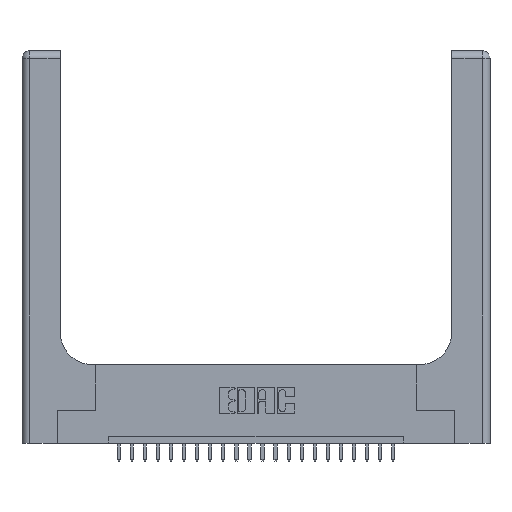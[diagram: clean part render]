
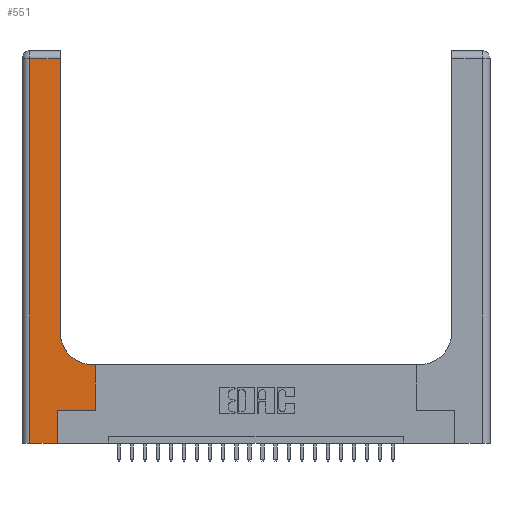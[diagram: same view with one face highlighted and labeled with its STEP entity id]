
A CAD part, top view. The second image highlights one B-rep face of the part: STEP entity #551.
In plain terms, the highlighted planar face has unit normal (0, 0, 1).
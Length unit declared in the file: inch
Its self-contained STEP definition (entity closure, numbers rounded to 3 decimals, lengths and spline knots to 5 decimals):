
#551 = ADVANCED_FACE ( 'NONE', ( #5901 ), #21168, .F. ) ;
#574 = ORIENTED_EDGE ( 'NONE', *, *, #9648, .T. ) ;
#747 = LINE ( 'NONE', #5997, #8378 ) ;
#786 = VECTOR ( 'NONE', #13788, 39.37008 ) ;
#1562 = EDGE_CURVE ( 'NONE', #21603, #2287, #7590, .T. ) ;
#2083 = VECTOR ( 'NONE', #13588, 39.37008 ) ;
#2287 = VERTEX_POINT ( 'NONE', #13245 ) ;
#2296 = DIRECTION ( 'NONE',  ( -1., 0., 0. ) ) ;
#2639 = CIRCLE ( 'NONE', #22379, 0.25 ) ;
#2671 = AXIS2_PLACEMENT_3D ( 'NONE', #17604, #11815, #23171 ) ;
#3718 = VERTEX_POINT ( 'NONE', #16368 ) ;
#3790 = VERTEX_POINT ( 'NONE', #22604 ) ;
#4397 = DIRECTION ( 'NONE',  ( 1., 0., 0. ) ) ;
#4873 = CARTESIAN_POINT ( 'NONE',  ( 0.06, 0., 0.37 ) ) ;
#4976 = ORIENTED_EDGE ( 'NONE', *, *, #11635, .T. ) ;
#5269 = CARTESIAN_POINT ( 'NONE',  ( 0.269, 0., 0.37 ) ) ;
#5380 = VECTOR ( 'NONE', #18151, 39.37008 ) ;
#5586 = EDGE_LOOP ( 'NONE', ( #23124, #16695, #574, #4976, #21441, #18248, #17871, #23331, #22186 ) ) ;
#5901 = FACE_OUTER_BOUND ( 'NONE', #5586, .T. ) ;
#5997 = CARTESIAN_POINT ( 'NONE',  ( 0., 2.94, 0.37 ) ) ;
#6001 = LINE ( 'NONE', #19905, #5380 ) ;
#6237 = EDGE_CURVE ( 'NONE', #6935, #3718, #2639, .T. ) ;
#6865 = VERTEX_POINT ( 'NONE', #20523 ) ;
#6935 = VERTEX_POINT ( 'NONE', #9733 ) ;
#7590 = LINE ( 'NONE', #5269, #19437 ) ;
#7670 = LINE ( 'NONE', #19273, #2083 ) ;
#8378 = VECTOR ( 'NONE', #2296, 39.37008 ) ;
#9127 = VECTOR ( 'NONE', #19043, 39.37008 ) ;
#9457 = CARTESIAN_POINT ( 'NONE',  ( 0.2915, 3., 0.37 ) ) ;
#9648 = EDGE_CURVE ( 'NONE', #6865, #11348, #6001, .T. ) ;
#9733 = CARTESIAN_POINT ( 'NONE',  ( 0.5415, 0.6, 0.37 ) ) ;
#11348 = VERTEX_POINT ( 'NONE', #4873 ) ;
#11635 = EDGE_CURVE ( 'NONE', #11348, #21603, #7670, .T. ) ;
#11815 = DIRECTION ( 'NONE',  ( 0., 0., -1. ) ) ;
#12939 = EDGE_CURVE ( 'NONE', #21963, #6935, #22930, .T. ) ;
#13245 = CARTESIAN_POINT ( 'NONE',  ( 0.269, 0.25, 0.37 ) ) ;
#13588 = DIRECTION ( 'NONE',  ( 1., 0., 0. ) ) ;
#13605 = CARTESIAN_POINT ( 'NONE',  ( 0.269, 0., 0.37 ) ) ;
#13788 = DIRECTION ( 'NONE',  ( -1., 0., 0. ) ) ;
#13867 = VECTOR ( 'NONE', #4397, 39.37008 ) ;
#13871 = CARTESIAN_POINT ( 'NONE',  ( 0.2915, 0.6, 0.37 ) ) ;
#13925 = VECTOR ( 'NONE', #23402, 39.37008 ) ;
#15688 = LINE ( 'NONE', #9457, #9127 ) ;
#15859 = EDGE_CURVE ( 'NONE', #3790, #21963, #22475, .T. ) ;
#16335 = CARTESIAN_POINT ( 'NONE',  ( 0.2915, 2.94, 0.37 ) ) ;
#16368 = CARTESIAN_POINT ( 'NONE',  ( 0.2915, 0.85, 0.37 ) ) ;
#16695 = ORIENTED_EDGE ( 'NONE', *, *, #18360, .T. ) ;
#17352 = VERTEX_POINT ( 'NONE', #16335 ) ;
#17411 = CARTESIAN_POINT ( 'NONE',  ( 0.5585, 0.25, 0.37 ) ) ;
#17604 = CARTESIAN_POINT ( 'NONE',  ( 0., 3., 0.37 ) ) ;
#17650 = DIRECTION ( 'NONE',  ( 1., 0., 0. ) ) ;
#17871 = ORIENTED_EDGE ( 'NONE', *, *, #15859, .T. ) ;
#17967 = DIRECTION ( 'NONE',  ( 0., 0., -1. ) ) ;
#18151 = DIRECTION ( 'NONE',  ( 0., -1., 0. ) ) ;
#18248 = ORIENTED_EDGE ( 'NONE', *, *, #22298, .T. ) ;
#18360 = EDGE_CURVE ( 'NONE', #17352, #6865, #747, .T. ) ;
#19043 = DIRECTION ( 'NONE',  ( 0., 1., 0. ) ) ;
#19177 = LINE ( 'NONE', #19669, #13867 ) ;
#19273 = CARTESIAN_POINT ( 'NONE',  ( 0., 0., 0.37 ) ) ;
#19437 = VECTOR ( 'NONE', #22316, 39.37008 ) ;
#19669 = CARTESIAN_POINT ( 'NONE',  ( 0.269, 0.25, 0.37 ) ) ;
#19905 = CARTESIAN_POINT ( 'NONE',  ( 0.06, 3., 0.37 ) ) ;
#20523 = CARTESIAN_POINT ( 'NONE',  ( 0.06, 2.94, 0.37 ) ) ;
#21168 = PLANE ( 'NONE',  #2671 ) ;
#21441 = ORIENTED_EDGE ( 'NONE', *, *, #1562, .T. ) ;
#21463 = CARTESIAN_POINT ( 'NONE',  ( 0.5415, 0.85, 0.37 ) ) ;
#21476 = EDGE_CURVE ( 'NONE', #3718, #17352, #15688, .T. ) ;
#21603 = VERTEX_POINT ( 'NONE', #13605 ) ;
#21963 = VERTEX_POINT ( 'NONE', #24319 ) ;
#22186 = ORIENTED_EDGE ( 'NONE', *, *, #6237, .T. ) ;
#22298 = EDGE_CURVE ( 'NONE', #2287, #3790, #19177, .T. ) ;
#22316 = DIRECTION ( 'NONE',  ( 0., 1., 0. ) ) ;
#22379 = AXIS2_PLACEMENT_3D ( 'NONE', #21463, #17967, #17650 ) ;
#22475 = LINE ( 'NONE', #17411, #13925 ) ;
#22604 = CARTESIAN_POINT ( 'NONE',  ( 0.5585, 0.25, 0.37 ) ) ;
#22930 = LINE ( 'NONE', #13871, #786 ) ;
#23124 = ORIENTED_EDGE ( 'NONE', *, *, #21476, .T. ) ;
#23171 = DIRECTION ( 'NONE',  ( -1., 0., 0. ) ) ;
#23331 = ORIENTED_EDGE ( 'NONE', *, *, #12939, .T. ) ;
#23402 = DIRECTION ( 'NONE',  ( 0., 1., 0. ) ) ;
#24319 = CARTESIAN_POINT ( 'NONE',  ( 0.5585, 0.6, 0.37 ) ) ;
